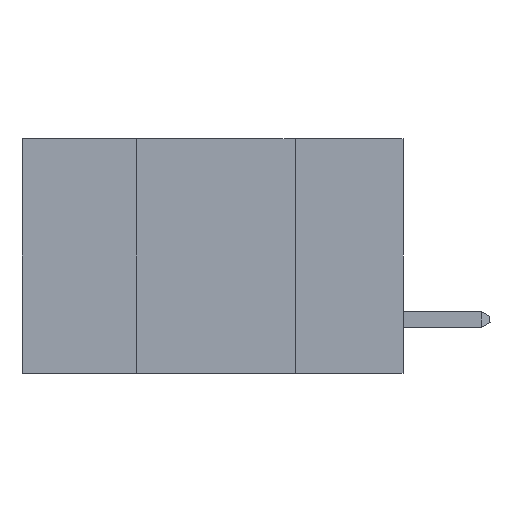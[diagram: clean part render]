
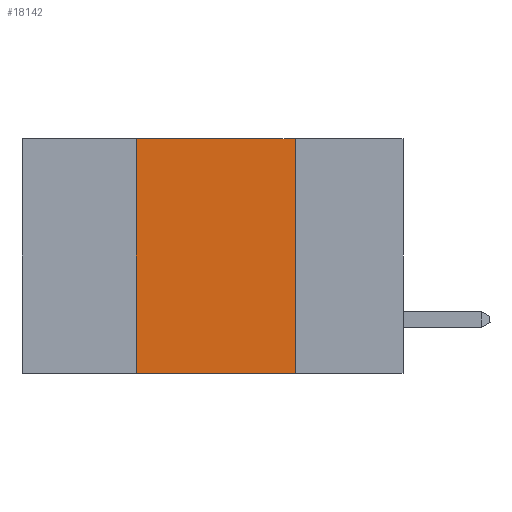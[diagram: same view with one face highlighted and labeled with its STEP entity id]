
A CAD part, left-side view. The second image highlights one B-rep face of the part: STEP entity #18142.
In plain terms, the highlighted planar face has unit normal (-1, 0, 0).
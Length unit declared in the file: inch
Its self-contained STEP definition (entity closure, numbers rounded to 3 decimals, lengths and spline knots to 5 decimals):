
#566 = FACE_OUTER_BOUND ( 'NONE', #9528, .T. ) ;
#1075 = VECTOR ( 'NONE', #17550, 39.37008 ) ;
#1121 = LINE ( 'NONE', #7111, #16598 ) ;
#1342 = CARTESIAN_POINT ( 'NONE',  ( 0., 0.17, 0. ) ) ;
#1562 = LINE ( 'NONE', #15999, #1075 ) ;
#2257 = ORIENTED_EDGE ( 'NONE', *, *, #17256, .F. ) ;
#3060 = PLANE ( 'NONE',  #17535 ) ;
#3236 = ORIENTED_EDGE ( 'NONE', *, *, #15088, .F. ) ;
#3593 = LINE ( 'NONE', #4398, #18489 ) ;
#3696 = VERTEX_POINT ( 'NONE', #7137 ) ;
#3701 = EDGE_CURVE ( 'NONE', #10068, #4999, #1121, .T. ) ;
#4398 = CARTESIAN_POINT ( 'NONE',  ( 0., 0.42, 0. ) ) ;
#4584 = CARTESIAN_POINT ( 'NONE',  ( 0., 0.6, 0. ) ) ;
#4999 = VERTEX_POINT ( 'NONE', #13793 ) ;
#5919 = DIRECTION ( 'NONE',  ( 0., 0., 1. ) ) ;
#6106 = DIRECTION ( 'NONE',  ( 0., 0., -1. ) ) ;
#7085 = DIRECTION ( 'NONE',  ( 0., 0., -1. ) ) ;
#7111 = CARTESIAN_POINT ( 'NONE',  ( 0., 0.17, 0. ) ) ;
#7137 = CARTESIAN_POINT ( 'NONE',  ( 0., 0.42, 0. ) ) ;
#7520 = VERTEX_POINT ( 'NONE', #16535 ) ;
#9528 = EDGE_LOOP ( 'NONE', ( #9827, #2257, #3236, #11220 ) ) ;
#9827 = ORIENTED_EDGE ( 'NONE', *, *, #3701, .F. ) ;
#10068 = VERTEX_POINT ( 'NONE', #1342 ) ;
#10873 = EDGE_CURVE ( 'NONE', #7520, #4999, #15975, .T. ) ;
#11220 = ORIENTED_EDGE ( 'NONE', *, *, #10873, .T. ) ;
#13793 = CARTESIAN_POINT ( 'NONE',  ( 0., 0.17, -0.37 ) ) ;
#14762 = DIRECTION ( 'NONE',  ( 0., -1., 0. ) ) ;
#15009 = DIRECTION ( 'NONE',  ( 1., 0., 0. ) ) ;
#15088 = EDGE_CURVE ( 'NONE', #7520, #3696, #3593, .T. ) ;
#15507 = VECTOR ( 'NONE', #14762, 39.37008 ) ;
#15975 = LINE ( 'NONE', #19122, #15507 ) ;
#15999 = CARTESIAN_POINT ( 'NONE',  ( 0., 0.6, 0. ) ) ;
#16535 = CARTESIAN_POINT ( 'NONE',  ( 0., 0.42, -0.37 ) ) ;
#16598 = VECTOR ( 'NONE', #7085, 39.37008 ) ;
#17256 = EDGE_CURVE ( 'NONE', #3696, #10068, #1562, .T. ) ;
#17535 = AXIS2_PLACEMENT_3D ( 'NONE', #4584, #15009, #6106 ) ;
#17550 = DIRECTION ( 'NONE',  ( 0., -1., 0. ) ) ;
#18142 = ADVANCED_FACE ( 'NONE', ( #566 ), #3060, .F. ) ;
#18489 = VECTOR ( 'NONE', #5919, 39.37008 ) ;
#19122 = CARTESIAN_POINT ( 'NONE',  ( 0., 0.6, -0.37 ) ) ;
